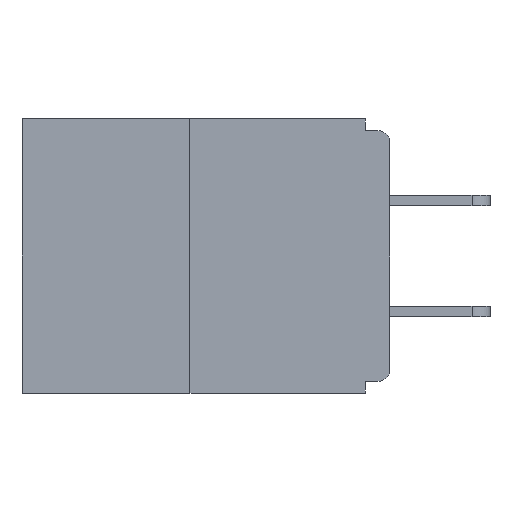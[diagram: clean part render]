
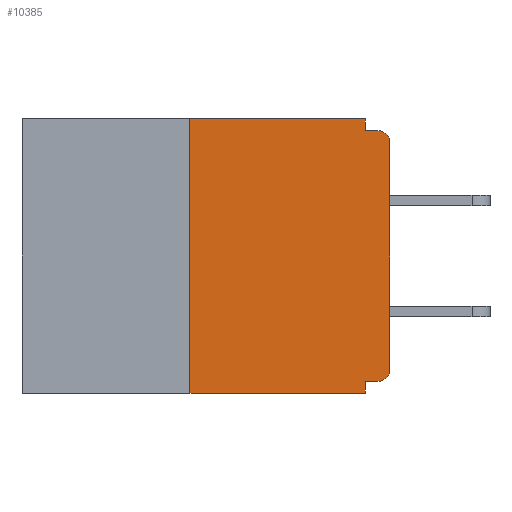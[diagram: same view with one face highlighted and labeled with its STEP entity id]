
A CAD part, left-side view. The second image highlights one B-rep face of the part: STEP entity #10385.
In plain terms, the highlighted planar face has unit normal (-1, 0, 0).
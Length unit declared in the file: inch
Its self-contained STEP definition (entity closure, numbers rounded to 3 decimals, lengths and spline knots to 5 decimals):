
#32 = CARTESIAN_POINT ( 'NONE',  ( 0., 0.46, 0. ) ) ;
#52 = CARTESIAN_POINT ( 'NONE',  ( 0., 0.25, -0.343 ) ) ;
#126 = VECTOR ( 'NONE', #9578, 39.37008 ) ;
#588 = CARTESIAN_POINT ( 'NONE',  ( 0., 0.031, -0.328 ) ) ;
#811 = LINE ( 'NONE', #10321, #4603 ) ;
#1069 = VERTEX_POINT ( 'NONE', #588 ) ;
#1443 = ORIENTED_EDGE ( 'NONE', *, *, #1979, .F. ) ;
#1447 = ORIENTED_EDGE ( 'NONE', *, *, #8348, .T. ) ;
#1979 = EDGE_CURVE ( 'NONE', #9394, #4101, #8582, .T. ) ;
#1997 = DIRECTION ( 'NONE',  ( 1., 0., 0. ) ) ;
#2060 = DIRECTION ( 'NONE',  ( -1., 0., 0. ) ) ;
#2152 = EDGE_CURVE ( 'NONE', #4021, #11917, #11680, .T. ) ;
#2165 = ORIENTED_EDGE ( 'NONE', *, *, #2152, .F. ) ;
#2754 = EDGE_CURVE ( 'NONE', #13061, #4021, #10180, .T. ) ;
#2909 = VECTOR ( 'NONE', #5207, 39.37008 ) ;
#2954 = ORIENTED_EDGE ( 'NONE', *, *, #2754, .F. ) ;
#3322 = AXIS2_PLACEMENT_3D ( 'NONE', #9929, #11882, #8817 ) ;
#3413 = LINE ( 'NONE', #9329, #5006 ) ;
#3508 = ORIENTED_EDGE ( 'NONE', *, *, #9866, .F. ) ;
#4021 = VERTEX_POINT ( 'NONE', #10296 ) ;
#4101 = VERTEX_POINT ( 'NONE', #11573 ) ;
#4197 = VERTEX_POINT ( 'NONE', #8929 ) ;
#4603 = VECTOR ( 'NONE', #10415, 39.37008 ) ;
#4914 = EDGE_CURVE ( 'NONE', #4197, #8297, #7051, .T. ) ;
#5006 = VECTOR ( 'NONE', #6311, 39.37008 ) ;
#5091 = AXIS2_PLACEMENT_3D ( 'NONE', #32, #1997, #5183 ) ;
#5103 = LINE ( 'NONE', #7736, #5242 ) ;
#5146 = DIRECTION ( 'NONE',  ( 0., -1., 0. ) ) ;
#5183 = DIRECTION ( 'NONE',  ( 0., 0., -1. ) ) ;
#5207 = DIRECTION ( 'NONE',  ( 0., 0., -1. ) ) ;
#5231 = ORIENTED_EDGE ( 'NONE', *, *, #12002, .T. ) ;
#5242 = VECTOR ( 'NONE', #5146, 39.37008 ) ;
#5931 = CARTESIAN_POINT ( 'NONE',  ( 0., 0.25, 0. ) ) ;
#5979 = DIRECTION ( 'NONE',  ( 0., 0., 1. ) ) ;
#6020 = EDGE_CURVE ( 'NONE', #7919, #1069, #3413, .T. ) ;
#6131 = CARTESIAN_POINT ( 'NONE',  ( 0., 0.031, -0.343 ) ) ;
#6311 = DIRECTION ( 'NONE',  ( 0., 1., 0. ) ) ;
#6867 = CARTESIAN_POINT ( 'NONE',  ( 0., 0., 0. ) ) ;
#7051 = LINE ( 'NONE', #6867, #7717 ) ;
#7090 = EDGE_CURVE ( 'NONE', #8297, #11917, #12876, .T. ) ;
#7183 = VERTEX_POINT ( 'NONE', #6131 ) ;
#7240 = CARTESIAN_POINT ( 'NONE',  ( 0., 0.031, 0. ) ) ;
#7512 = AXIS2_PLACEMENT_3D ( 'NONE', #11185, #2060, #13100 ) ;
#7615 = CARTESIAN_POINT ( 'NONE',  ( 0., 0.015, -0.015 ) ) ;
#7717 = VECTOR ( 'NONE', #5979, 39.37008 ) ;
#7736 = CARTESIAN_POINT ( 'NONE',  ( 0., 0.46, -0.343 ) ) ;
#7754 = CARTESIAN_POINT ( 'NONE',  ( 0., 0.46, 0. ) ) ;
#7919 = VERTEX_POINT ( 'NONE', #8288 ) ;
#7959 = VECTOR ( 'NONE', #9944, 39.37008 ) ;
#8019 = CARTESIAN_POINT ( 'NONE',  ( 0., 0., -0.03 ) ) ;
#8156 = LINE ( 'NONE', #7754, #9106 ) ;
#8288 = CARTESIAN_POINT ( 'NONE',  ( 0., 0.015, -0.328 ) ) ;
#8297 = VERTEX_POINT ( 'NONE', #8019 ) ;
#8348 = EDGE_CURVE ( 'NONE', #9394, #7183, #5103, .T. ) ;
#8582 = LINE ( 'NONE', #5931, #7959 ) ;
#8817 = DIRECTION ( 'NONE',  ( 0., 0., -1. ) ) ;
#8899 = DIRECTION ( 'NONE',  ( 0., -1., 0. ) ) ;
#8929 = CARTESIAN_POINT ( 'NONE',  ( 0., 0., -0.313 ) ) ;
#9106 = VECTOR ( 'NONE', #8899, 39.37008 ) ;
#9329 = CARTESIAN_POINT ( 'NONE',  ( 0., 0., -0.328 ) ) ;
#9394 = VERTEX_POINT ( 'NONE', #52 ) ;
#9578 = DIRECTION ( 'NONE',  ( 0., -1., 0. ) ) ;
#9758 = ORIENTED_EDGE ( 'NONE', *, *, #4914, .T. ) ;
#9823 = ORIENTED_EDGE ( 'NONE', *, *, #7090, .T. ) ;
#9866 = EDGE_CURVE ( 'NONE', #1069, #7183, #811, .T. ) ;
#9929 = CARTESIAN_POINT ( 'NONE',  ( 0., 0.015, -0.313 ) ) ;
#9944 = DIRECTION ( 'NONE',  ( 0., 0., 1. ) ) ;
#10180 = LINE ( 'NONE', #11257, #2909 ) ;
#10296 = CARTESIAN_POINT ( 'NONE',  ( 0., 0.031, -0.015 ) ) ;
#10321 = CARTESIAN_POINT ( 'NONE',  ( 0., 0.031, -0.343 ) ) ;
#10385 = ADVANCED_FACE ( 'NONE', ( #11367 ), #12145, .F. ) ;
#10415 = DIRECTION ( 'NONE',  ( 0., 0., -1. ) ) ;
#10739 = ORIENTED_EDGE ( 'NONE', *, *, #6020, .F. ) ;
#11185 = CARTESIAN_POINT ( 'NONE',  ( 0., 0.015, -0.03 ) ) ;
#11257 = CARTESIAN_POINT ( 'NONE',  ( 0., 0.031, 0. ) ) ;
#11367 = FACE_OUTER_BOUND ( 'NONE', #12099, .T. ) ;
#11411 = ORIENTED_EDGE ( 'NONE', *, *, #12070, .F. ) ;
#11573 = CARTESIAN_POINT ( 'NONE',  ( 0., 0.25, 0. ) ) ;
#11680 = LINE ( 'NONE', #12708, #126 ) ;
#11882 = DIRECTION ( 'NONE',  ( -1., 0., 0. ) ) ;
#11917 = VERTEX_POINT ( 'NONE', #7615 ) ;
#12002 = EDGE_CURVE ( 'NONE', #7919, #4197, #12114, .T. ) ;
#12070 = EDGE_CURVE ( 'NONE', #4101, #13061, #8156, .T. ) ;
#12099 = EDGE_LOOP ( 'NONE', ( #11411, #1443, #1447, #3508, #10739, #5231, #9758, #9823, #2165, #2954 ) ) ;
#12114 = CIRCLE ( 'NONE', #3322, 0.015 ) ;
#12145 = PLANE ( 'NONE',  #5091 ) ;
#12708 = CARTESIAN_POINT ( 'NONE',  ( 0., 0., -0.015 ) ) ;
#12876 = CIRCLE ( 'NONE', #7512, 0.015 ) ;
#13061 = VERTEX_POINT ( 'NONE', #7240 ) ;
#13100 = DIRECTION ( 'NONE',  ( 0., 0., -1. ) ) ;
